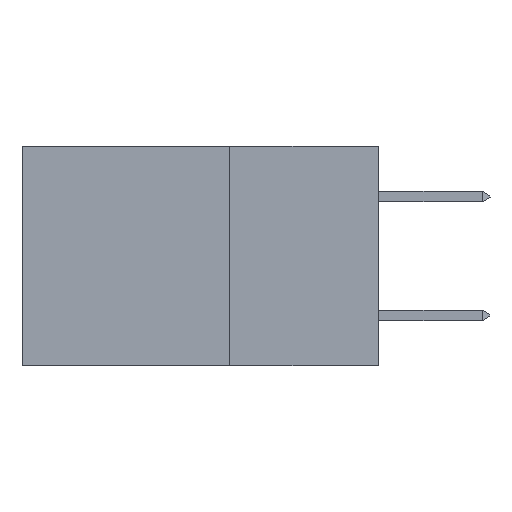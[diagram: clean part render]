
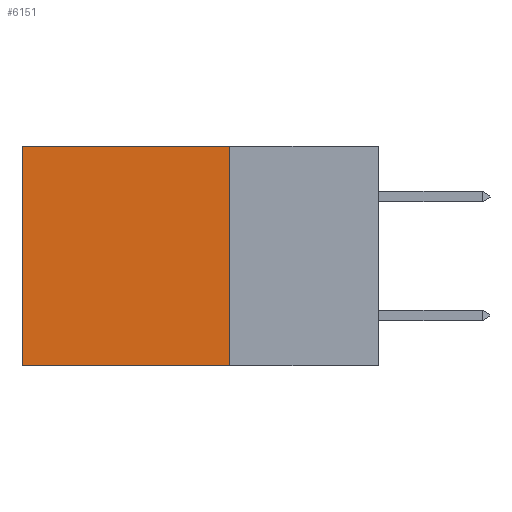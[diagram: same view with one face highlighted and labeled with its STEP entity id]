
A CAD part, left-side view. The second image highlights one B-rep face of the part: STEP entity #6151.
In plain terms, the highlighted planar face has unit normal (-1, 0, 0).
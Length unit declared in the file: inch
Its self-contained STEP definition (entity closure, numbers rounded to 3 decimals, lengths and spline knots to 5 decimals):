
#862 = CARTESIAN_POINT ( 'NONE',  ( 0.298, 0.25, 0. ) ) ;
#1409 = LINE ( 'NONE', #862, #8596 ) ;
#1670 = DIRECTION ( 'NONE',  ( 0., 0., -1. ) ) ;
#1868 = VERTEX_POINT ( 'NONE', #8407 ) ;
#2264 = DIRECTION ( 'NONE',  ( 0., 1., 0. ) ) ;
#2335 = EDGE_CURVE ( 'NONE', #4061, #7680, #4325, .T. ) ;
#2465 = AXIS2_PLACEMENT_3D ( 'NONE', #8619, #4095, #7725 ) ;
#2700 = ORIENTED_EDGE ( 'NONE', *, *, #10638, .F. ) ;
#3049 = CARTESIAN_POINT ( 'NONE',  ( 0.298, 0.25, 0. ) ) ;
#3069 = CARTESIAN_POINT ( 'NONE',  ( 0.298, 0.25, 0. ) ) ;
#3423 = VECTOR ( 'NONE', #2264, 39.37008 ) ;
#4061 = VERTEX_POINT ( 'NONE', #3069 ) ;
#4095 = DIRECTION ( 'NONE',  ( 1., 0., 0. ) ) ;
#4325 = LINE ( 'NONE', #3049, #9716 ) ;
#5354 = CARTESIAN_POINT ( 'NONE',  ( 0.298, 0.6, 0. ) ) ;
#5483 = ORIENTED_EDGE ( 'NONE', *, *, #2335, .T. ) ;
#5962 = LINE ( 'NONE', #8147, #10370 ) ;
#6151 = ADVANCED_FACE ( 'NONE', ( #6217 ), #6681, .F. ) ;
#6217 = FACE_OUTER_BOUND ( 'NONE', #11141, .T. ) ;
#6392 = DIRECTION ( 'NONE',  ( 0., 0., -1. ) ) ;
#6594 = EDGE_CURVE ( 'NONE', #1868, #9019, #8148, .T. ) ;
#6681 = PLANE ( 'NONE',  #2465 ) ;
#6812 = CARTESIAN_POINT ( 'NONE',  ( 0.298, 0.6, -0.37 ) ) ;
#7680 = VERTEX_POINT ( 'NONE', #5354 ) ;
#7725 = DIRECTION ( 'NONE',  ( 0., 0., -1. ) ) ;
#8147 = CARTESIAN_POINT ( 'NONE',  ( 0.298, 0.6, 0. ) ) ;
#8148 = LINE ( 'NONE', #9297, #3423 ) ;
#8407 = CARTESIAN_POINT ( 'NONE',  ( 0.298, 0.25, -0.37 ) ) ;
#8445 = ORIENTED_EDGE ( 'NONE', *, *, #6594, .F. ) ;
#8596 = VECTOR ( 'NONE', #1670, 39.37008 ) ;
#8619 = CARTESIAN_POINT ( 'NONE',  ( 0.298, 0.25, 0. ) ) ;
#9019 = VERTEX_POINT ( 'NONE', #6812 ) ;
#9228 = DIRECTION ( 'NONE',  ( 0., 1., 0. ) ) ;
#9297 = CARTESIAN_POINT ( 'NONE',  ( 0.298, 0.25, -0.37 ) ) ;
#9594 = ORIENTED_EDGE ( 'NONE', *, *, #10702, .T. ) ;
#9716 = VECTOR ( 'NONE', #9228, 39.37008 ) ;
#10370 = VECTOR ( 'NONE', #6392, 39.37008 ) ;
#10638 = EDGE_CURVE ( 'NONE', #4061, #1868, #1409, .T. ) ;
#10702 = EDGE_CURVE ( 'NONE', #7680, #9019, #5962, .T. ) ;
#11141 = EDGE_LOOP ( 'NONE', ( #9594, #8445, #2700, #5483 ) ) ;
